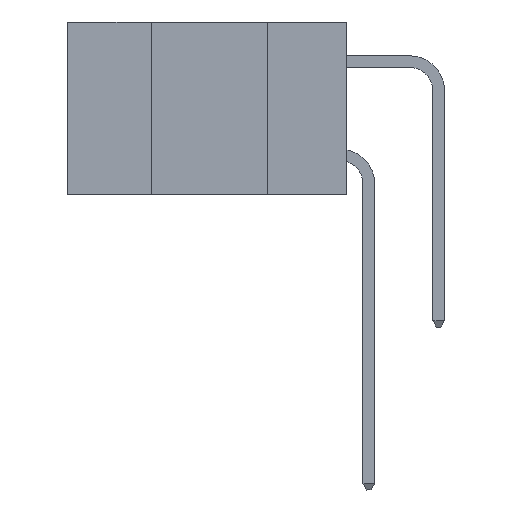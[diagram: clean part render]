
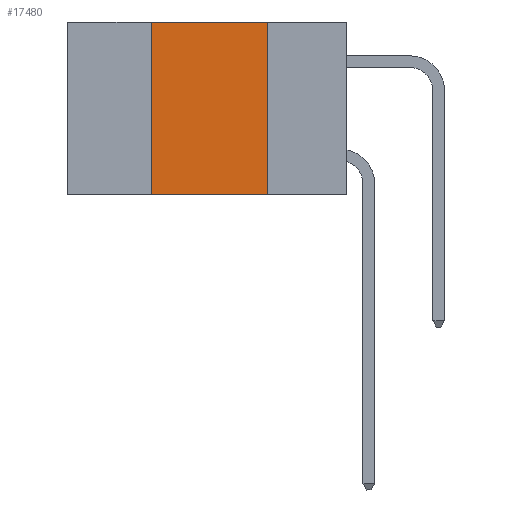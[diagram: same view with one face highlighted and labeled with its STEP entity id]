
A CAD part, left-side view. The second image highlights one B-rep face of the part: STEP entity #17480.
In plain terms, the highlighted planar face has unit normal (-1, 0, 0).
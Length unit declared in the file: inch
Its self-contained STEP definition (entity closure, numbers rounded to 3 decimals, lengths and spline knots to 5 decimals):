
#160 = EDGE_CURVE ( 'NONE', #12199, #4993, #21785, .T. ) ;
#209 = VECTOR ( 'NONE', #10763, 39.37008 ) ;
#218 = CARTESIAN_POINT ( 'NONE',  ( 0., 0.17, 0. ) ) ;
#755 = ORIENTED_EDGE ( 'NONE', *, *, #15320, .F. ) ;
#1500 = CARTESIAN_POINT ( 'NONE',  ( 0., 0.42, 0. ) ) ;
#2086 = CARTESIAN_POINT ( 'NONE',  ( 0., 0.6, -0.37 ) ) ;
#2758 = EDGE_LOOP ( 'NONE', ( #18149, #10079, #755, #16003 ) ) ;
#4609 = PLANE ( 'NONE',  #16438 ) ;
#4952 = LINE ( 'NONE', #11183, #17965 ) ;
#4993 = VERTEX_POINT ( 'NONE', #22328 ) ;
#7065 = VERTEX_POINT ( 'NONE', #19310 ) ;
#8208 = DIRECTION ( 'NONE',  ( 0., 0., -1. ) ) ;
#9103 = LINE ( 'NONE', #14346, #209 ) ;
#9164 = DIRECTION ( 'NONE',  ( 0., -1., 0. ) ) ;
#9814 = EDGE_CURVE ( 'NONE', #7065, #4993, #9928, .T. ) ;
#9928 = LINE ( 'NONE', #2086, #14665 ) ;
#10079 = ORIENTED_EDGE ( 'NONE', *, *, #21124, .F. ) ;
#10763 = DIRECTION ( 'NONE',  ( 0., 0., 1. ) ) ;
#11183 = CARTESIAN_POINT ( 'NONE',  ( 0., 0.6, 0. ) ) ;
#11284 = DIRECTION ( 'NONE',  ( 0., 0., -1. ) ) ;
#11398 = VERTEX_POINT ( 'NONE', #1500 ) ;
#12199 = VERTEX_POINT ( 'NONE', #218 ) ;
#13474 = FACE_OUTER_BOUND ( 'NONE', #2758, .T. ) ;
#14346 = CARTESIAN_POINT ( 'NONE',  ( 0., 0.42, 0. ) ) ;
#14665 = VECTOR ( 'NONE', #9164, 39.37008 ) ;
#14772 = DIRECTION ( 'NONE',  ( 0., -1., 0. ) ) ;
#15320 = EDGE_CURVE ( 'NONE', #7065, #11398, #9103, .T. ) ;
#16003 = ORIENTED_EDGE ( 'NONE', *, *, #9814, .T. ) ;
#16351 = CARTESIAN_POINT ( 'NONE',  ( 0., 0.17, 0. ) ) ;
#16438 = AXIS2_PLACEMENT_3D ( 'NONE', #17045, #18757, #8208 ) ;
#17045 = CARTESIAN_POINT ( 'NONE',  ( 0., 0.6, 0. ) ) ;
#17480 = ADVANCED_FACE ( 'NONE', ( #13474 ), #4609, .F. ) ;
#17965 = VECTOR ( 'NONE', #14772, 39.37008 ) ;
#18149 = ORIENTED_EDGE ( 'NONE', *, *, #160, .F. ) ;
#18757 = DIRECTION ( 'NONE',  ( 1., 0., 0. ) ) ;
#19310 = CARTESIAN_POINT ( 'NONE',  ( 0., 0.42, -0.37 ) ) ;
#21124 = EDGE_CURVE ( 'NONE', #11398, #12199, #4952, .T. ) ;
#21214 = VECTOR ( 'NONE', #11284, 39.37008 ) ;
#21785 = LINE ( 'NONE', #16351, #21214 ) ;
#22328 = CARTESIAN_POINT ( 'NONE',  ( 0., 0.17, -0.37 ) ) ;
